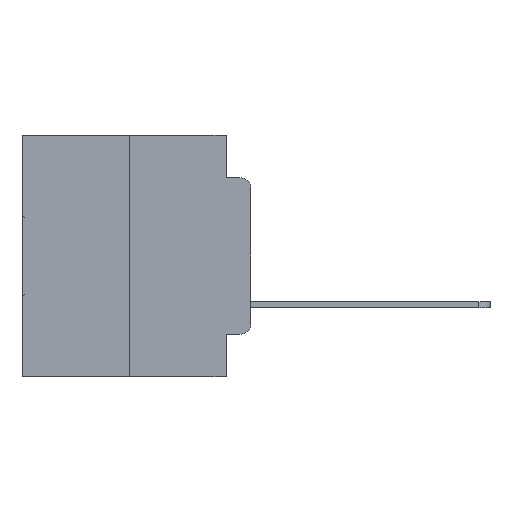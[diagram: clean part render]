
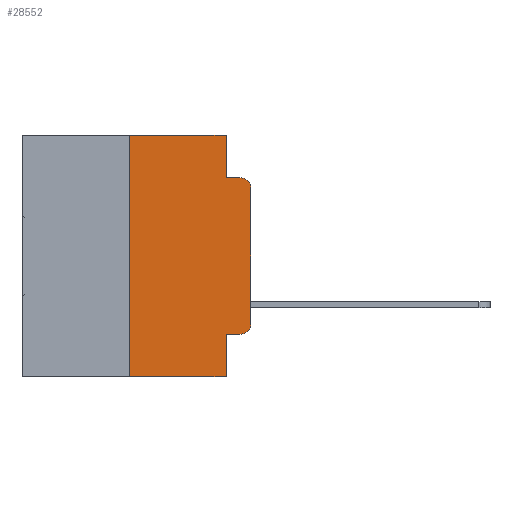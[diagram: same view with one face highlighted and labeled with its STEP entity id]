
A CAD part, left-side view. The second image highlights one B-rep face of the part: STEP entity #28552.
In plain terms, the highlighted planar face has unit normal (-1, 0, 0).
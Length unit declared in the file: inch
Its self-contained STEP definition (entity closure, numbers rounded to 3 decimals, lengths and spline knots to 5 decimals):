
#69 = LINE ( 'NONE', #28347, #25173 ) ;
#1005 = AXIS2_PLACEMENT_3D ( 'NONE', #7840, #24528, #10309 ) ;
#1304 = ORIENTED_EDGE ( 'NONE', *, *, #8485, .F. ) ;
#1587 = EDGE_CURVE ( 'NONE', #19011, #7613, #23203, .T. ) ;
#3046 = CARTESIAN_POINT ( 'NONE',  ( 0., 0.02, -0.4115 ) ) ;
#3176 = DIRECTION ( 'NONE',  ( 0., -1., 0. ) ) ;
#3408 = EDGE_CURVE ( 'NONE', #20705, #15789, #25200, .T. ) ;
#3422 = CARTESIAN_POINT ( 'NONE',  ( 0., 0., -0.3915 ) ) ;
#4793 = VECTOR ( 'NONE', #13243, 39.37008 ) ;
#5191 = CARTESIAN_POINT ( 'NONE',  ( 0., 0.051, -0.0885 ) ) ;
#5643 = EDGE_CURVE ( 'NONE', #23351, #22625, #24025, .T. ) ;
#6044 = ORIENTED_EDGE ( 'NONE', *, *, #8585, .F. ) ;
#6110 = CARTESIAN_POINT ( 'NONE',  ( 0., 0.02, -0.1085 ) ) ;
#6141 = FACE_OUTER_BOUND ( 'NONE', #17356, .T. ) ;
#6185 = EDGE_CURVE ( 'NONE', #11356, #8874, #19585, .T. ) ;
#6464 = ORIENTED_EDGE ( 'NONE', *, *, #3408, .T. ) ;
#7613 = VERTEX_POINT ( 'NONE', #3046 ) ;
#7840 = CARTESIAN_POINT ( 'NONE',  ( 0., 0.02, -0.3915 ) ) ;
#8126 = LINE ( 'NONE', #26864, #14602 ) ;
#8133 = PLANE ( 'NONE',  #8412 ) ;
#8333 = EDGE_CURVE ( 'NONE', #7613, #14668, #14966, .T. ) ;
#8412 = AXIS2_PLACEMENT_3D ( 'NONE', #13035, #29364, #15461 ) ;
#8430 = DIRECTION ( 'NONE',  ( 0., 0., -1. ) ) ;
#8485 = EDGE_CURVE ( 'NONE', #19011, #15789, #23854, .T. ) ;
#8585 = EDGE_CURVE ( 'NONE', #20619, #8874, #8126, .T. ) ;
#8618 = DIRECTION ( 'NONE',  ( 0., 0., -1. ) ) ;
#8874 = VERTEX_POINT ( 'NONE', #11506 ) ;
#9537 = ORIENTED_EDGE ( 'NONE', *, *, #30902, .T. ) ;
#9733 = VECTOR ( 'NONE', #18056, 39.37008 ) ;
#9897 = VECTOR ( 'NONE', #26457, 39.37008 ) ;
#10309 = DIRECTION ( 'NONE',  ( 0., 0., -1. ) ) ;
#11204 = VECTOR ( 'NONE', #29473, 39.37008 ) ;
#11356 = VERTEX_POINT ( 'NONE', #27538 ) ;
#11506 = CARTESIAN_POINT ( 'NONE',  ( 0., 0.02, -0.0885 ) ) ;
#11869 = ORIENTED_EDGE ( 'NONE', *, *, #8333, .T. ) ;
#11939 = DIRECTION ( 'NONE',  ( 0., 0., 1. ) ) ;
#12638 = VECTOR ( 'NONE', #3176, 39.37008 ) ;
#13035 = CARTESIAN_POINT ( 'NONE',  ( 0., 0.473, 0. ) ) ;
#13243 = DIRECTION ( 'NONE',  ( 0., -1., 0. ) ) ;
#14057 = VECTOR ( 'NONE', #8430, 39.37008 ) ;
#14101 = ORIENTED_EDGE ( 'NONE', *, *, #16442, .F. ) ;
#14602 = VECTOR ( 'NONE', #17602, 39.37008 ) ;
#14668 = VERTEX_POINT ( 'NONE', #3422 ) ;
#14966 = CIRCLE ( 'NONE', #1005, 0.02 ) ;
#15221 = EDGE_CURVE ( 'NONE', #20705, #23351, #69, .T. ) ;
#15405 = CARTESIAN_POINT ( 'NONE',  ( 0., 0.473, -0.5 ) ) ;
#15461 = DIRECTION ( 'NONE',  ( 0., 0., -1. ) ) ;
#15648 = CARTESIAN_POINT ( 'NONE',  ( 0., 0.051, -0.4115 ) ) ;
#15789 = VERTEX_POINT ( 'NONE', #24427 ) ;
#15982 = ORIENTED_EDGE ( 'NONE', *, *, #1587, .T. ) ;
#16344 = ORIENTED_EDGE ( 'NONE', *, *, #15221, .F. ) ;
#16442 = EDGE_CURVE ( 'NONE', #22625, #20619, #20360, .T. ) ;
#17070 = LINE ( 'NONE', #30908, #9897 ) ;
#17356 = EDGE_LOOP ( 'NONE', ( #9537, #17453, #6044, #14101, #21940, #16344, #6464, #1304, #15982, #11869 ) ) ;
#17453 = ORIENTED_EDGE ( 'NONE', *, *, #6185, .T. ) ;
#17602 = DIRECTION ( 'NONE',  ( 0., -1., 0. ) ) ;
#17971 = CARTESIAN_POINT ( 'NONE',  ( 0., 0.051, 0. ) ) ;
#18056 = DIRECTION ( 'NONE',  ( 0., -1., 0. ) ) ;
#18871 = CARTESIAN_POINT ( 'NONE',  ( 0., 0.051, 0. ) ) ;
#19011 = VERTEX_POINT ( 'NONE', #28115 ) ;
#19585 = CIRCLE ( 'NONE', #19843, 0.02 ) ;
#19634 = CARTESIAN_POINT ( 'NONE',  ( 0., 0.25, 0. ) ) ;
#19843 = AXIS2_PLACEMENT_3D ( 'NONE', #6110, #22985, #8618 ) ;
#20360 = LINE ( 'NONE', #22818, #14057 ) ;
#20619 = VERTEX_POINT ( 'NONE', #5191 ) ;
#20705 = VERTEX_POINT ( 'NONE', #29300 ) ;
#21940 = ORIENTED_EDGE ( 'NONE', *, *, #5643, .F. ) ;
#22625 = VERTEX_POINT ( 'NONE', #18871 ) ;
#22818 = CARTESIAN_POINT ( 'NONE',  ( 0., 0.051, 0. ) ) ;
#22985 = DIRECTION ( 'NONE',  ( -1., 0., 0. ) ) ;
#23203 = LINE ( 'NONE', #15648, #9733 ) ;
#23351 = VERTEX_POINT ( 'NONE', #19634 ) ;
#23854 = LINE ( 'NONE', #17971, #11204 ) ;
#24025 = LINE ( 'NONE', #29541, #4793 ) ;
#24427 = CARTESIAN_POINT ( 'NONE',  ( 0., 0.051, -0.5 ) ) ;
#24528 = DIRECTION ( 'NONE',  ( -1., 0., 0. ) ) ;
#25173 = VECTOR ( 'NONE', #11939, 39.37008 ) ;
#25200 = LINE ( 'NONE', #15405, #12638 ) ;
#26457 = DIRECTION ( 'NONE',  ( 0., 0., 1. ) ) ;
#26864 = CARTESIAN_POINT ( 'NONE',  ( 0., 0.051, -0.0885 ) ) ;
#27538 = CARTESIAN_POINT ( 'NONE',  ( 0., 0., -0.1085 ) ) ;
#28115 = CARTESIAN_POINT ( 'NONE',  ( 0., 0.051, -0.4115 ) ) ;
#28347 = CARTESIAN_POINT ( 'NONE',  ( 0., 0.25, 0. ) ) ;
#28552 = ADVANCED_FACE ( 'NONE', ( #6141 ), #8133, .F. ) ;
#29300 = CARTESIAN_POINT ( 'NONE',  ( 0., 0.25, -0.5 ) ) ;
#29364 = DIRECTION ( 'NONE',  ( 1., 0., 0. ) ) ;
#29473 = DIRECTION ( 'NONE',  ( 0., 0., -1. ) ) ;
#29541 = CARTESIAN_POINT ( 'NONE',  ( 0., 0.473, 0. ) ) ;
#30902 = EDGE_CURVE ( 'NONE', #14668, #11356, #17070, .T. ) ;
#30908 = CARTESIAN_POINT ( 'NONE',  ( 0., 0., 0. ) ) ;
